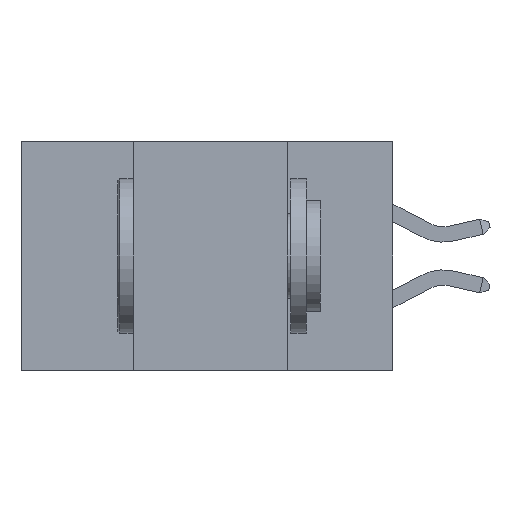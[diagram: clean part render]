
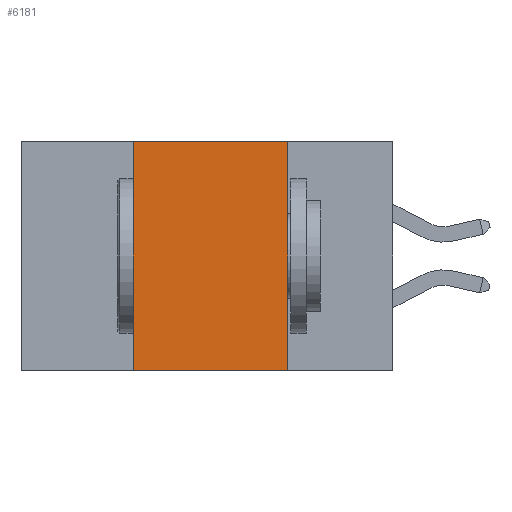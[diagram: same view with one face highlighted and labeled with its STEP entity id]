
A CAD part, left-side view. The second image highlights one B-rep face of the part: STEP entity #6181.
In plain terms, the highlighted planar face has unit normal (-1, 0, 0).
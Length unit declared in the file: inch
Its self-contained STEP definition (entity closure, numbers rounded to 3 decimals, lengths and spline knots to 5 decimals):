
#293 = CARTESIAN_POINT ( 'NONE',  ( 0., 0.42, 0. ) ) ;
#942 = CARTESIAN_POINT ( 'NONE',  ( 0., 0.17, -0.37 ) ) ;
#1907 = CARTESIAN_POINT ( 'NONE',  ( 0., 0.6, 0. ) ) ;
#2169 = LINE ( 'NONE', #2987, #25353 ) ;
#2987 = CARTESIAN_POINT ( 'NONE',  ( 0., 0.6, 0. ) ) ;
#3656 = CARTESIAN_POINT ( 'NONE',  ( 0., 0.6, -0.37 ) ) ;
#4428 = EDGE_CURVE ( 'NONE', #5060, #10668, #6649, .T. ) ;
#4451 = CARTESIAN_POINT ( 'NONE',  ( 0., 0.42, 0. ) ) ;
#4583 = EDGE_CURVE ( 'NONE', #26968, #5060, #2169, .T. ) ;
#4849 = CARTESIAN_POINT ( 'NONE',  ( 0., 0.42, -0.37 ) ) ;
#5018 = VECTOR ( 'NONE', #26178, 39.37008 ) ;
#5060 = VERTEX_POINT ( 'NONE', #24184 ) ;
#6075 = FACE_OUTER_BOUND ( 'NONE', #21631, .T. ) ;
#6181 = ADVANCED_FACE ( 'NONE', ( #6075 ), #12588, .F. ) ;
#6343 = DIRECTION ( 'NONE',  ( 0., 0., -1. ) ) ;
#6649 = LINE ( 'NONE', #11165, #23297 ) ;
#7023 = ORIENTED_EDGE ( 'NONE', *, *, #4583, .F. ) ;
#9372 = ORIENTED_EDGE ( 'NONE', *, *, #4428, .F. ) ;
#9879 = VECTOR ( 'NONE', #14126, 39.37008 ) ;
#10668 = VERTEX_POINT ( 'NONE', #942 ) ;
#11039 = AXIS2_PLACEMENT_3D ( 'NONE', #1907, #15070, #6343 ) ;
#11165 = CARTESIAN_POINT ( 'NONE',  ( 0., 0.17, 0. ) ) ;
#12588 = PLANE ( 'NONE',  #11039 ) ;
#14126 = DIRECTION ( 'NONE',  ( 0., -1., 0. ) ) ;
#15070 = DIRECTION ( 'NONE',  ( 1., 0., 0. ) ) ;
#15583 = LINE ( 'NONE', #4451, #5018 ) ;
#16636 = VERTEX_POINT ( 'NONE', #4849 ) ;
#20570 = ORIENTED_EDGE ( 'NONE', *, *, #23356, .T. ) ;
#21090 = LINE ( 'NONE', #3656, #9879 ) ;
#21631 = EDGE_LOOP ( 'NONE', ( #9372, #7023, #25252, #20570 ) ) ;
#23297 = VECTOR ( 'NONE', #24041, 39.37008 ) ;
#23356 = EDGE_CURVE ( 'NONE', #16636, #10668, #21090, .T. ) ;
#24041 = DIRECTION ( 'NONE',  ( 0., 0., -1. ) ) ;
#24184 = CARTESIAN_POINT ( 'NONE',  ( 0., 0.17, 0. ) ) ;
#24505 = DIRECTION ( 'NONE',  ( 0., -1., 0. ) ) ;
#25252 = ORIENTED_EDGE ( 'NONE', *, *, #25700, .F. ) ;
#25353 = VECTOR ( 'NONE', #24505, 39.37008 ) ;
#25700 = EDGE_CURVE ( 'NONE', #16636, #26968, #15583, .T. ) ;
#26178 = DIRECTION ( 'NONE',  ( 0., 0., 1. ) ) ;
#26968 = VERTEX_POINT ( 'NONE', #293 ) ;
